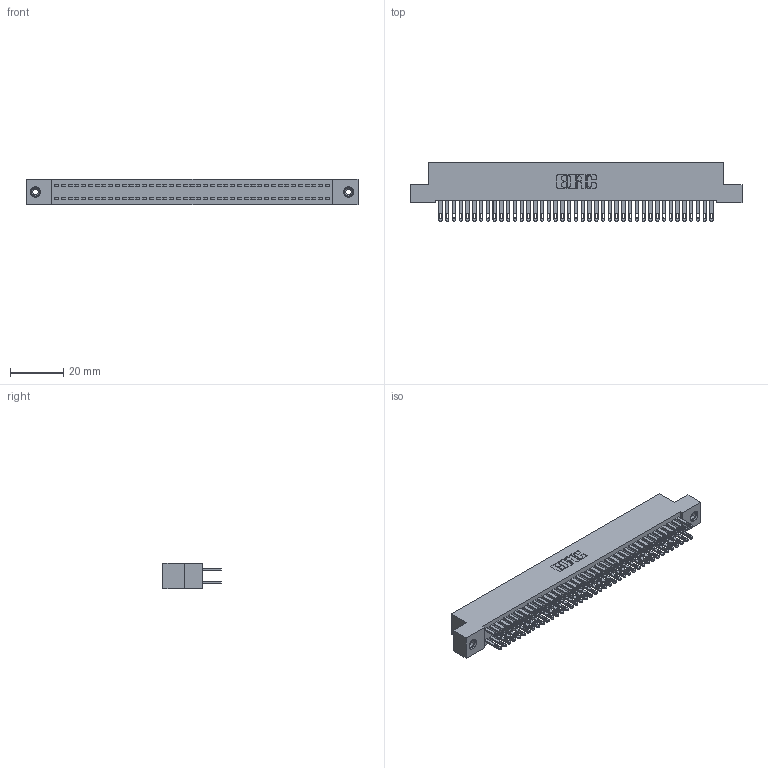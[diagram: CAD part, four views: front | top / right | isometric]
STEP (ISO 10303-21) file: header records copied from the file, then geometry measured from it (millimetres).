
FILE_DESCRIPTION (( 'STEP AP203' ), '1' );
FILE_NAME ('342-082-500-208.STEP', '2019-10-04T11:57:44', ( '' ), ( '' ), 'SwSTEP 2.0', 'SolidWorks 2016', '' );
FILE_SCHEMA (( 'CONFIG_CONTROL_DESIGN' ));
Length unit declared in the file: inch
Products named in the file (4): 345-292-001_345-293-100; 345-250-001_345-250-003-102; 342-082-500-208; 342 Part_TI
Assembly tree (85 placements, depth 2):
  342-082-500-208
    342 Part_TI
    345-292-001_345-293-100  x82
    345-250-001_345-250-003-102  x2
Bounding box: 124.46 x 21.85 x 9.4 mm (x, y, z)
Volume: 11422.9 mm3; surface area: 19364.3 mm2
Topology: 85 solids, 85 shells, 4106 faces, 12489 edges, 8318 vertices
Faces by surface type: plane 2558, cylinder 1532, cone 12, torus 4
Entity records: 27490 total; most frequent: CARTESIAN_POINT 4537, ORIENTED_EDGE 4466, DIRECTION 3911, EDGE_CURVE 2233, LINE 2081, VECTOR 2081, VERTEX_POINT 1484, AXIS2_PLACEMENT_3D 915
